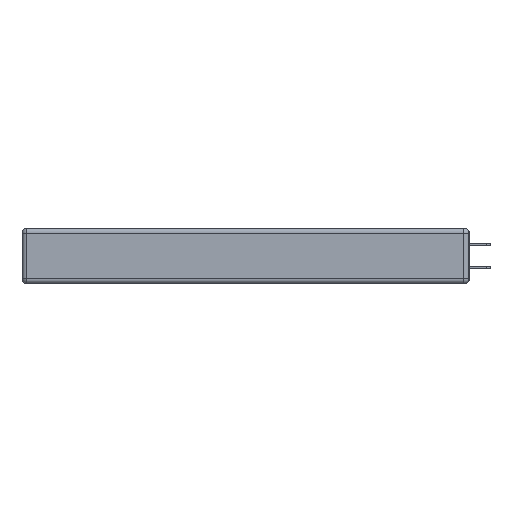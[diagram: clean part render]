
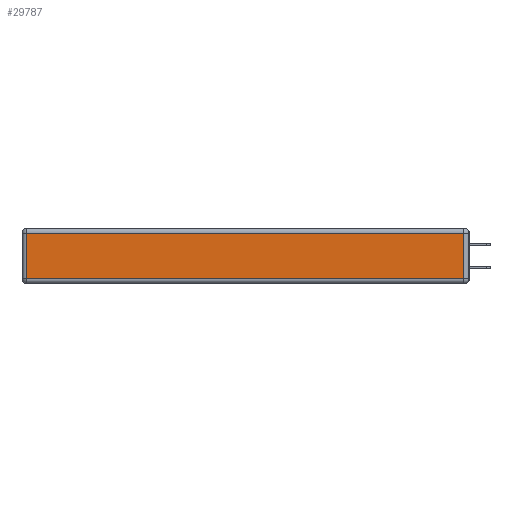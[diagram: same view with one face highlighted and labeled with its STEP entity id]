
A CAD part, left-side view. The second image highlights one B-rep face of the part: STEP entity #29787.
In plain terms, the highlighted planar face has unit normal (-1, 0, 0).
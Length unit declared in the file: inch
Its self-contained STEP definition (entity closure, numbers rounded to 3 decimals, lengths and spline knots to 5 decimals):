
#185 = CARTESIAN_POINT ( 'NONE',  ( 0., 2.72, -0.313 ) ) ;
#2672 = VECTOR ( 'NONE', #7077, 39.37008 ) ;
#2709 = EDGE_CURVE ( 'NONE', #32881, #15486, #19584, .T. ) ;
#2855 = LINE ( 'NONE', #23074, #20018 ) ;
#3104 = AXIS2_PLACEMENT_3D ( 'NONE', #18398, #26207, #28836 ) ;
#3771 = CARTESIAN_POINT ( 'NONE',  ( 0., 0., -0.313 ) ) ;
#4585 = ORIENTED_EDGE ( 'NONE', *, *, #2709, .T. ) ;
#6590 = CARTESIAN_POINT ( 'NONE',  ( 0., 0.03, -0.343 ) ) ;
#6685 = FACE_OUTER_BOUND ( 'NONE', #32496, .T. ) ;
#7077 = DIRECTION ( 'NONE',  ( 0., -1., 0. ) ) ;
#9313 = EDGE_CURVE ( 'NONE', #15486, #11260, #2855, .T. ) ;
#9338 = CARTESIAN_POINT ( 'NONE',  ( 0., 0.03, -0.03 ) ) ;
#11260 = VERTEX_POINT ( 'NONE', #185 ) ;
#11725 = LINE ( 'NONE', #6590, #28048 ) ;
#12765 = CARTESIAN_POINT ( 'NONE',  ( 0., 2.72, -0.03 ) ) ;
#14120 = CARTESIAN_POINT ( 'NONE',  ( 0., 0.03, -0.313 ) ) ;
#15301 = DIRECTION ( 'NONE',  ( 0., 1., 0. ) ) ;
#15339 = ORIENTED_EDGE ( 'NONE', *, *, #16200, .T. ) ;
#15486 = VERTEX_POINT ( 'NONE', #12765 ) ;
#16200 = EDGE_CURVE ( 'NONE', #11260, #22822, #18167, .T. ) ;
#17243 = ORIENTED_EDGE ( 'NONE', *, *, #33339, .T. ) ;
#18012 = ORIENTED_EDGE ( 'NONE', *, *, #9313, .T. ) ;
#18167 = LINE ( 'NONE', #3771, #2672 ) ;
#18398 = CARTESIAN_POINT ( 'NONE',  ( 0., 0., -0.343 ) ) ;
#19584 = LINE ( 'NONE', #30971, #30116 ) ;
#20018 = VECTOR ( 'NONE', #33551, 39.37008 ) ;
#22822 = VERTEX_POINT ( 'NONE', #14120 ) ;
#23074 = CARTESIAN_POINT ( 'NONE',  ( 0., 2.72, -0.343 ) ) ;
#23646 = PLANE ( 'NONE',  #3104 ) ;
#26207 = DIRECTION ( 'NONE',  ( -1., 0., 0. ) ) ;
#28048 = VECTOR ( 'NONE', #29349, 39.37008 ) ;
#28836 = DIRECTION ( 'NONE',  ( 0., 0., 1. ) ) ;
#29349 = DIRECTION ( 'NONE',  ( 0., 0., 1. ) ) ;
#29787 = ADVANCED_FACE ( 'NONE', ( #6685 ), #23646, .T. ) ;
#30116 = VECTOR ( 'NONE', #15301, 39.37008 ) ;
#30971 = CARTESIAN_POINT ( 'NONE',  ( 0., 2.75, -0.03 ) ) ;
#32496 = EDGE_LOOP ( 'NONE', ( #15339, #17243, #4585, #18012 ) ) ;
#32881 = VERTEX_POINT ( 'NONE', #9338 ) ;
#33339 = EDGE_CURVE ( 'NONE', #22822, #32881, #11725, .T. ) ;
#33551 = DIRECTION ( 'NONE',  ( 0., 0., -1. ) ) ;
